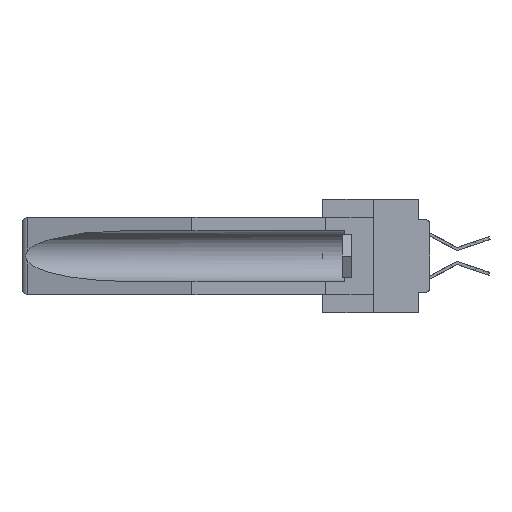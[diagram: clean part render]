
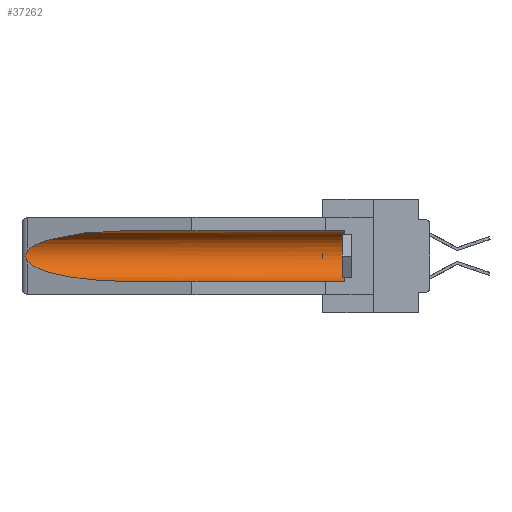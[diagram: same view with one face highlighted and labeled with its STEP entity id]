
A CAD part, left-side view. The second image highlights one B-rep face of the part: STEP entity #37262.
In plain terms, the highlighted cylindrical face has radius 2.857 mm (diameter 5.715 mm), a partial arc.
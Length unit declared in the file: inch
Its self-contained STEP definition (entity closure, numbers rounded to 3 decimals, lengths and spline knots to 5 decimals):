
#1095 = ORIENTED_EDGE ( 'NONE', *, *, #25880, .T. ) ;
#1185 = EDGE_CURVE ( 'NONE', #14551, #24089, #28680, .T. ) ;
#1590 = DIRECTION ( 'NONE',  ( 0., 0., 1. ) ) ;
#1807 = CARTESIAN_POINT ( 'NONE',  ( 0.2675, 1.53308, -0.16763 ) ) ;
#2662 = VECTOR ( 'NONE', #26830, 39.37008 ) ;
#3103 = CARTESIAN_POINT ( 'NONE',  ( 0.21114, 1.30732, -0.284 ) ) ;
#3919 = LINE ( 'NONE', #5398, #36742 ) ;
#5010 = EDGE_CURVE ( 'NONE', #5239, #14551, #13330, .T. ) ;
#5239 = VERTEX_POINT ( 'NONE', #6509 ) ;
#5367 = ORIENTED_EDGE ( 'NONE', *, *, #1185, .T. ) ;
#5398 = CARTESIAN_POINT ( 'NONE',  ( 0.155, -0.30754, -0.284 ) ) ;
#6247 = ORIENTED_EDGE ( 'NONE', *, *, #27218, .T. ) ;
#6509 = CARTESIAN_POINT ( 'NONE',  ( 0.26537, 1.52718, -0.14972 ) ) ;
#6607 = AXIS2_PLACEMENT_3D ( 'NONE', #11082, #26698, #26556 ) ;
#7802 = AXIS2_PLACEMENT_3D ( 'NONE', #27596, #23985, #1590 ) ;
#7896 = CARTESIAN_POINT ( 'NONE',  ( 0.155, 1.07973, -0.059 ) ) ;
#8302 = CARTESIAN_POINT ( 'NONE',  ( 0.26654, 1.53092, -0.15636 ) ) ;
#10099 = CIRCLE ( 'NONE', #6607, 0.1125 ) ;
#10291 = ORIENTED_EDGE ( 'NONE', *, *, #37929, .F. ) ;
#11082 = CARTESIAN_POINT ( 'NONE',  ( 0.155, 0.126, -0.1715 ) ) ;
#11092 = CARTESIAN_POINT ( 'NONE',  ( 0.26655, 1.53094, -0.18657 ) ) ;
#11207 = VERTEX_POINT ( 'NONE', #20625 ) ;
#12370 = CARTESIAN_POINT ( 'NONE',  ( 0.25451, 1.48313, -0.09465 ) ) ;
#13330 = B_SPLINE_CURVE_WITH_KNOTS ( 'NONE', 3,
 ( #31737, #25787, #8302, #23909, #1807, #28106, #30396, #11092, #24064, #33595 ),
 .UNSPECIFIED., .F., .F.,
 ( 4, 2, 2, 2, 4 ),
 ( 0., 0.00029, 0.00058, 0.00087, 0.00117 ),
 .UNSPECIFIED. ) ;
#13924 = CYLINDRICAL_SURFACE ( 'NONE', #7802, 0.1125 ) ;
#14551 = VERTEX_POINT ( 'NONE', #24040 ) ;
#15419 = CARTESIAN_POINT ( 'NONE',  ( 0.155, 1.07973, -0.059 ) ) ;
#15601 = CARTESIAN_POINT ( 'NONE',  ( 0.25451, 1.48313, -0.24835 ) ) ;
#15862 = CARTESIAN_POINT ( 'NONE',  ( 0.155, 1.07973, -0.284 ) ) ;
#15937 = CARTESIAN_POINT ( 'NONE',  ( 0.155, 0.126, -0.059 ) ) ;
#17900 = CARTESIAN_POINT ( 'NONE',  ( 0.155, 1.07973, -0.284 ) ) ;
#20625 = CARTESIAN_POINT ( 'NONE',  ( 0.155, 0.126, -0.284 ) ) ;
#20683 = CARTESIAN_POINT ( 'NONE',  ( 0.155, -0.30754, -0.059 ) ) ;
#21277 = DIRECTION ( 'NONE',  ( 0., 1., 0. ) ) ;
#21874 = CARTESIAN_POINT ( 'NONE',  ( 0.21114, 1.30732, -0.059 ) ) ;
#22079 = LINE ( 'NONE', #20683, #2662 ) ;
#23909 = CARTESIAN_POINT ( 'NONE',  ( 0.2673, 1.5327, -0.16383 ) ) ;
#23985 = DIRECTION ( 'NONE',  ( 0., 1., 0. ) ) ;
#24040 = CARTESIAN_POINT ( 'NONE',  ( 0.26537, 1.52718, -0.19328 ) ) ;
#24064 = CARTESIAN_POINT ( 'NONE',  ( 0.26597, 1.5296, -0.19026 ) ) ;
#24089 = VERTEX_POINT ( 'NONE', #17900 ) ;
#25787 = CARTESIAN_POINT ( 'NONE',  ( 0.26597, 1.52961, -0.15275 ) ) ;
#25880 = EDGE_CURVE ( 'NONE', #11207, #39118, #10099, .T. ) ;
#26556 = DIRECTION ( 'NONE',  ( 0., 0., 1. ) ) ;
#26698 = DIRECTION ( 'NONE',  ( 0., -1., 0. ) ) ;
#26811 = EDGE_CURVE ( 'NONE', #37837, #5239, #36549, .T. ) ;
#26830 = DIRECTION ( 'NONE',  ( 0., 1., 0. ) ) ;
#27218 = EDGE_CURVE ( 'NONE', #39118, #37837, #22079, .T. ) ;
#27596 = CARTESIAN_POINT ( 'NONE',  ( 0.155, -0.30754, -0.1715 ) ) ;
#28106 = CARTESIAN_POINT ( 'NONE',  ( 0.2675, 1.53308, -0.17534 ) ) ;
#28282 = CARTESIAN_POINT ( 'NONE',  ( 0.26537, 1.52718, -0.19328 ) ) ;
#28680 =( BOUNDED_CURVE ( )  B_SPLINE_CURVE ( 3, ( #28282, #15601, #3103, #15862 ),
 .UNSPECIFIED., .F., .F. ) 
 B_SPLINE_CURVE_WITH_KNOTS ( ( 4, 4 ),
 ( 0.1948, 1.5708 ),
 .UNSPECIFIED. ) 
 CURVE ( )  GEOMETRIC_REPRESENTATION_ITEM ( )  RATIONAL_B_SPLINE_CURVE ( ( 1., 0.848, 0.848, 1. ) ) 
 REPRESENTATION_ITEM ( '' )  );
#30334 = FACE_OUTER_BOUND ( 'NONE', #38164, .T. ) ;
#30396 = CARTESIAN_POINT ( 'NONE',  ( 0.2673, 1.53269, -0.17917 ) ) ;
#31737 = CARTESIAN_POINT ( 'NONE',  ( 0.26537, 1.52718, -0.14972 ) ) ;
#33595 = CARTESIAN_POINT ( 'NONE',  ( 0.26537, 1.52718, -0.19328 ) ) ;
#35018 = ORIENTED_EDGE ( 'NONE', *, *, #26811, .T. ) ;
#36549 =( BOUNDED_CURVE ( )  B_SPLINE_CURVE ( 3, ( #15419, #21874, #12370, #37896 ),
 .UNSPECIFIED., .F., .F. ) 
 B_SPLINE_CURVE_WITH_KNOTS ( ( 4, 4 ),
 ( 4.71239, 6.08839 ),
 .UNSPECIFIED. ) 
 CURVE ( )  GEOMETRIC_REPRESENTATION_ITEM ( )  RATIONAL_B_SPLINE_CURVE ( ( 1., 0.848, 0.848, 1. ) ) 
 REPRESENTATION_ITEM ( '' )  );
#36742 = VECTOR ( 'NONE', #21277, 39.37008 ) ;
#37262 = ADVANCED_FACE ( 'NONE', ( #30334 ), #13924, .F. ) ;
#37837 = VERTEX_POINT ( 'NONE', #7896 ) ;
#37896 = CARTESIAN_POINT ( 'NONE',  ( 0.26537, 1.52718, -0.14972 ) ) ;
#37929 = EDGE_CURVE ( 'NONE', #11207, #24089, #3919, .T. ) ;
#38164 = EDGE_LOOP ( 'NONE', ( #35018, #39219, #5367, #10291, #1095, #6247 ) ) ;
#39118 = VERTEX_POINT ( 'NONE', #15937 ) ;
#39219 = ORIENTED_EDGE ( 'NONE', *, *, #5010, .T. ) ;
